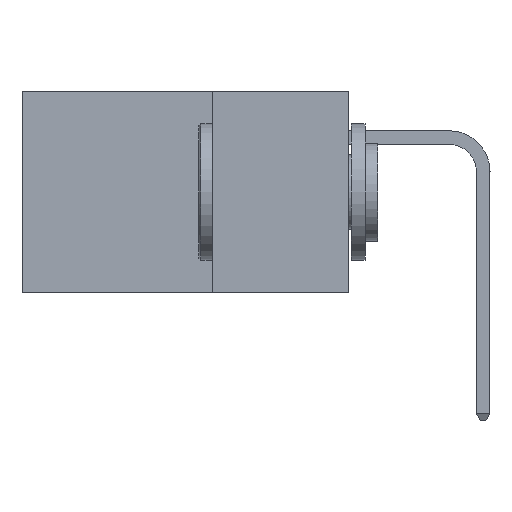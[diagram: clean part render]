
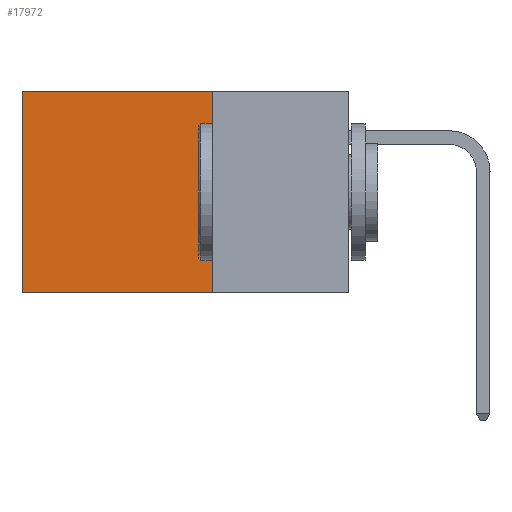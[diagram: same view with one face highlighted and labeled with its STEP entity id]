
A CAD part, left-side view. The second image highlights one B-rep face of the part: STEP entity #17972.
In plain terms, the highlighted planar face has unit normal (-1, 0, 0).
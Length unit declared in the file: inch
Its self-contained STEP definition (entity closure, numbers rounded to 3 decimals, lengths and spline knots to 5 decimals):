
#116 = LINE ( 'NONE', #1130, #8902 ) ;
#877 = DIRECTION ( 'NONE',  ( 0., 0., -1. ) ) ;
#1130 = CARTESIAN_POINT ( 'NONE',  ( 0.2875, 0.25, -0.37 ) ) ;
#2124 = DIRECTION ( 'NONE',  ( 0., 0., -1. ) ) ;
#6482 = VECTOR ( 'NONE', #2124, 39.37008 ) ;
#8902 = VECTOR ( 'NONE', #8994, 39.37008 ) ;
#8994 = DIRECTION ( 'NONE',  ( 0., 1., 0. ) ) ;
#10008 = CARTESIAN_POINT ( 'NONE',  ( 0.2875, 0.25, 0. ) ) ;
#11607 = PLANE ( 'NONE',  #38452 ) ;
#12587 = CARTESIAN_POINT ( 'NONE',  ( 0.2875, 0.25, 0. ) ) ;
#13575 = ORIENTED_EDGE ( 'NONE', *, *, #40737, .F. ) ;
#13595 = EDGE_CURVE ( 'NONE', #30703, #37723, #43424, .T. ) ;
#14578 = CARTESIAN_POINT ( 'NONE',  ( 0.2875, 0.25, 0. ) ) ;
#16526 = VERTEX_POINT ( 'NONE', #38406 ) ;
#17091 = VERTEX_POINT ( 'NONE', #14578 ) ;
#17972 = ADVANCED_FACE ( 'NONE', ( #27991 ), #11607, .F. ) ;
#18059 = VECTOR ( 'NONE', #24142, 39.37008 ) ;
#21248 = CARTESIAN_POINT ( 'NONE',  ( 0.2875, 0.6, -0.37 ) ) ;
#22092 = CARTESIAN_POINT ( 'NONE',  ( 0.2875, 0.6, 0. ) ) ;
#22578 = EDGE_LOOP ( 'NONE', ( #29346, #13575, #22994, #30386 ) ) ;
#22994 = ORIENTED_EDGE ( 'NONE', *, *, #25061, .F. ) ;
#24142 = DIRECTION ( 'NONE',  ( 0., 1., 0. ) ) ;
#25061 = EDGE_CURVE ( 'NONE', #17091, #16526, #39270, .T. ) ;
#27991 = FACE_OUTER_BOUND ( 'NONE', #22578, .T. ) ;
#29346 = ORIENTED_EDGE ( 'NONE', *, *, #13595, .T. ) ;
#30386 = ORIENTED_EDGE ( 'NONE', *, *, #43042, .T. ) ;
#30703 = VERTEX_POINT ( 'NONE', #41972 ) ;
#32733 = DIRECTION ( 'NONE',  ( 1., 0., 0. ) ) ;
#34554 = LINE ( 'NONE', #10008, #18059 ) ;
#36087 = CARTESIAN_POINT ( 'NONE',  ( 0.2875, 0.25, 0. ) ) ;
#37723 = VERTEX_POINT ( 'NONE', #21248 ) ;
#38406 = CARTESIAN_POINT ( 'NONE',  ( 0.2875, 0.25, -0.37 ) ) ;
#38452 = AXIS2_PLACEMENT_3D ( 'NONE', #36087, #32733, #39579 ) ;
#39270 = LINE ( 'NONE', #12587, #6482 ) ;
#39579 = DIRECTION ( 'NONE',  ( 0., 0., -1. ) ) ;
#40737 = EDGE_CURVE ( 'NONE', #16526, #37723, #116, .T. ) ;
#41972 = CARTESIAN_POINT ( 'NONE',  ( 0.2875, 0.6, 0. ) ) ;
#42847 = VECTOR ( 'NONE', #877, 39.37008 ) ;
#43042 = EDGE_CURVE ( 'NONE', #17091, #30703, #34554, .T. ) ;
#43424 = LINE ( 'NONE', #22092, #42847 ) ;
